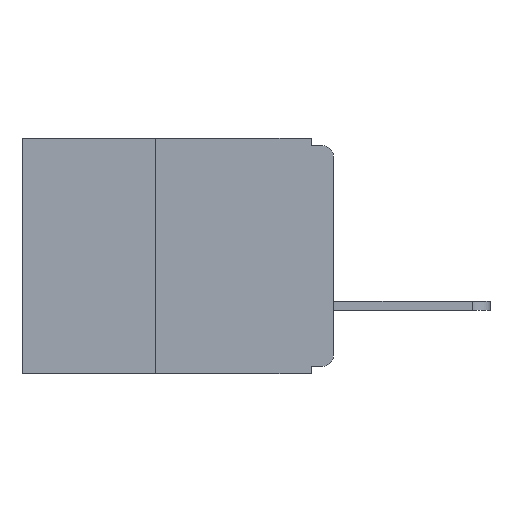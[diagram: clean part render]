
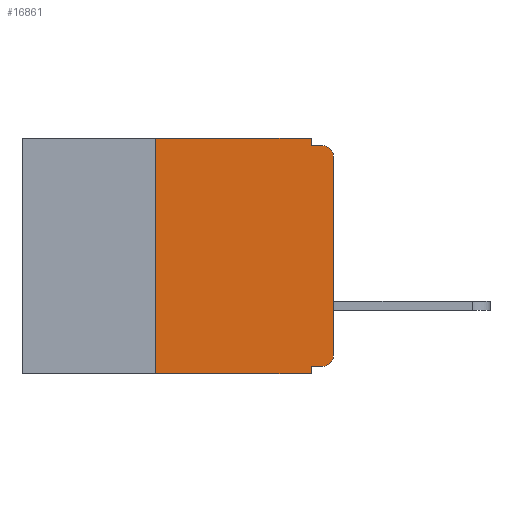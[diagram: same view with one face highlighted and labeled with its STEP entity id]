
A CAD part, left-side view. The second image highlights one B-rep face of the part: STEP entity #16861.
In plain terms, the highlighted planar face has unit normal (-1, 0, 0).
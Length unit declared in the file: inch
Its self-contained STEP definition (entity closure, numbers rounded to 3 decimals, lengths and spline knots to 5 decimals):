
#45 = VECTOR ( 'NONE', #27336, 39.37008 ) ;
#394 = LINE ( 'NONE', #14253, #25278 ) ;
#1584 = DIRECTION ( 'NONE',  ( -1., 0., 0. ) ) ;
#1774 = DIRECTION ( 'NONE',  ( 0., 0., -1. ) ) ;
#2253 = EDGE_CURVE ( 'NONE', #2499, #28693, #10858, .T. ) ;
#2499 = VERTEX_POINT ( 'NONE', #31117 ) ;
#2769 = ORIENTED_EDGE ( 'NONE', *, *, #25413, .F. ) ;
#3501 = EDGE_CURVE ( 'NONE', #3810, #13264, #32054, .T. ) ;
#3810 = VERTEX_POINT ( 'NONE', #10244 ) ;
#4235 = VECTOR ( 'NONE', #5954, 39.37008 ) ;
#4997 = EDGE_CURVE ( 'NONE', #6449, #27971, #8319, .T. ) ;
#5179 = DIRECTION ( 'NONE',  ( 0., 0., -1. ) ) ;
#5525 = VERTEX_POINT ( 'NONE', #7777 ) ;
#5798 = LINE ( 'NONE', #30689, #4235 ) ;
#5883 = VECTOR ( 'NONE', #29792, 39.37008 ) ;
#5890 = ORIENTED_EDGE ( 'NONE', *, *, #31076, .T. ) ;
#5954 = DIRECTION ( 'NONE',  ( 0., -1., 0. ) ) ;
#6387 = CARTESIAN_POINT ( 'NONE',  ( 0., 0.031, -0.32 ) ) ;
#6449 = VERTEX_POINT ( 'NONE', #12491 ) ;
#6662 = LINE ( 'NONE', #32130, #45 ) ;
#7396 = CARTESIAN_POINT ( 'NONE',  ( 0., 0.031, 0. ) ) ;
#7405 = CIRCLE ( 'NONE', #26067, 0.015 ) ;
#7777 = CARTESIAN_POINT ( 'NONE',  ( 0., 0., -0.025 ) ) ;
#8319 = LINE ( 'NONE', #17223, #27370 ) ;
#9638 = DIRECTION ( 'NONE',  ( 1., 0., 0. ) ) ;
#9754 = ORIENTED_EDGE ( 'NONE', *, *, #31320, .T. ) ;
#9923 = CARTESIAN_POINT ( 'NONE',  ( 0., 0., -0.32 ) ) ;
#10244 = CARTESIAN_POINT ( 'NONE',  ( 0., 0.015, -0.32 ) ) ;
#10620 = CARTESIAN_POINT ( 'NONE',  ( 0., 0.25, -0.33 ) ) ;
#10858 = LINE ( 'NONE', #10620, #11629 ) ;
#11154 = ORIENTED_EDGE ( 'NONE', *, *, #20580, .F. ) ;
#11629 = VECTOR ( 'NONE', #25019, 39.37008 ) ;
#12491 = CARTESIAN_POINT ( 'NONE',  ( 0., 0.031, -0.01 ) ) ;
#12742 = ORIENTED_EDGE ( 'NONE', *, *, #14357, .F. ) ;
#13264 = VERTEX_POINT ( 'NONE', #29554 ) ;
#13761 = VERTEX_POINT ( 'NONE', #23527 ) ;
#14253 = CARTESIAN_POINT ( 'NONE',  ( 0., 0.031, 0. ) ) ;
#14357 = EDGE_CURVE ( 'NONE', #28693, #24472, #26047, .T. ) ;
#16403 = AXIS2_PLACEMENT_3D ( 'NONE', #22287, #21528, #21459 ) ;
#16525 = CARTESIAN_POINT ( 'NONE',  ( 0., 0.015, -0.025 ) ) ;
#16800 = DIRECTION ( 'NONE',  ( 0., -1., 0. ) ) ;
#16861 = ADVANCED_FACE ( 'NONE', ( #27414 ), #24502, .F. ) ;
#16951 = LINE ( 'NONE', #22530, #29330 ) ;
#16992 = EDGE_CURVE ( 'NONE', #18438, #13761, #16951, .T. ) ;
#17223 = CARTESIAN_POINT ( 'NONE',  ( 0., 0., -0.01 ) ) ;
#18200 = ORIENTED_EDGE ( 'NONE', *, *, #26290, .T. ) ;
#18438 = VERTEX_POINT ( 'NONE', #6387 ) ;
#18564 = DIRECTION ( 'NONE',  ( 0., -1., 0. ) ) ;
#19021 = DIRECTION ( 'NONE',  ( 0., 0., -1. ) ) ;
#19156 = LINE ( 'NONE', #9923, #5883 ) ;
#19455 = VECTOR ( 'NONE', #18564, 39.37008 ) ;
#19558 = CARTESIAN_POINT ( 'NONE',  ( 0., 0.437, 0. ) ) ;
#19686 = CARTESIAN_POINT ( 'NONE',  ( 0., 0.015, -0.01 ) ) ;
#20580 = EDGE_CURVE ( 'NONE', #24472, #6449, #394, .T. ) ;
#20897 = ORIENTED_EDGE ( 'NONE', *, *, #2253, .F. ) ;
#21260 = ORIENTED_EDGE ( 'NONE', *, *, #4997, .F. ) ;
#21459 = DIRECTION ( 'NONE',  ( 0., 0., -1. ) ) ;
#21528 = DIRECTION ( 'NONE',  ( -1., 0., 0. ) ) ;
#22287 = CARTESIAN_POINT ( 'NONE',  ( 0., 0.015, -0.305 ) ) ;
#22487 = EDGE_LOOP ( 'NONE', ( #9754, #5890, #21260, #11154, #12742, #20897, #18200, #26409, #2769, #31190 ) ) ;
#22530 = CARTESIAN_POINT ( 'NONE',  ( 0., 0.031, -0.33 ) ) ;
#23384 = CARTESIAN_POINT ( 'NONE',  ( 0., 0.437, 0. ) ) ;
#23527 = CARTESIAN_POINT ( 'NONE',  ( 0., 0.031, -0.33 ) ) ;
#24472 = VERTEX_POINT ( 'NONE', #7396 ) ;
#24502 = PLANE ( 'NONE',  #28897 ) ;
#25019 = DIRECTION ( 'NONE',  ( 0., 0., 1. ) ) ;
#25030 = CARTESIAN_POINT ( 'NONE',  ( 0., 0.25, 0. ) ) ;
#25278 = VECTOR ( 'NONE', #1774, 39.37008 ) ;
#25413 = EDGE_CURVE ( 'NONE', #3810, #18438, #19156, .T. ) ;
#26047 = LINE ( 'NONE', #23384, #19455 ) ;
#26067 = AXIS2_PLACEMENT_3D ( 'NONE', #16525, #1584, #19021 ) ;
#26290 = EDGE_CURVE ( 'NONE', #2499, #13761, #5798, .T. ) ;
#26409 = ORIENTED_EDGE ( 'NONE', *, *, #16992, .F. ) ;
#27020 = DIRECTION ( 'NONE',  ( 0., 0., -1. ) ) ;
#27336 = DIRECTION ( 'NONE',  ( 0., 0., 1. ) ) ;
#27370 = VECTOR ( 'NONE', #16800, 39.37008 ) ;
#27414 = FACE_OUTER_BOUND ( 'NONE', #22487, .T. ) ;
#27971 = VERTEX_POINT ( 'NONE', #19686 ) ;
#28693 = VERTEX_POINT ( 'NONE', #25030 ) ;
#28897 = AXIS2_PLACEMENT_3D ( 'NONE', #19558, #9638, #27020 ) ;
#29330 = VECTOR ( 'NONE', #5179, 39.37008 ) ;
#29554 = CARTESIAN_POINT ( 'NONE',  ( 0., 0., -0.305 ) ) ;
#29792 = DIRECTION ( 'NONE',  ( 0., 1., 0. ) ) ;
#30689 = CARTESIAN_POINT ( 'NONE',  ( 0., 0.437, -0.33 ) ) ;
#31076 = EDGE_CURVE ( 'NONE', #5525, #27971, #7405, .T. ) ;
#31117 = CARTESIAN_POINT ( 'NONE',  ( 0., 0.25, -0.33 ) ) ;
#31190 = ORIENTED_EDGE ( 'NONE', *, *, #3501, .T. ) ;
#31320 = EDGE_CURVE ( 'NONE', #13264, #5525, #6662, .T. ) ;
#32054 = CIRCLE ( 'NONE', #16403, 0.015 ) ;
#32130 = CARTESIAN_POINT ( 'NONE',  ( 0., 0., 0. ) ) ;
